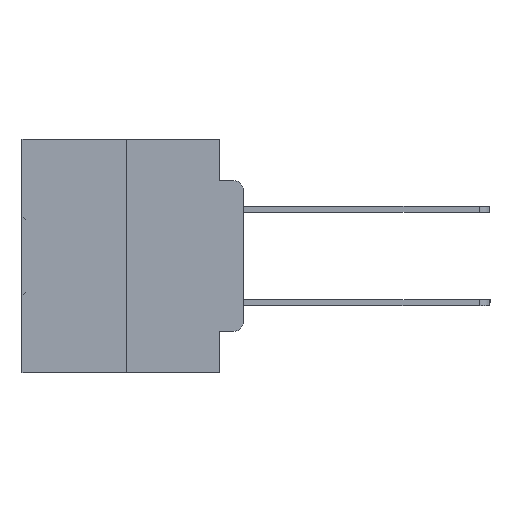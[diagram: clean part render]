
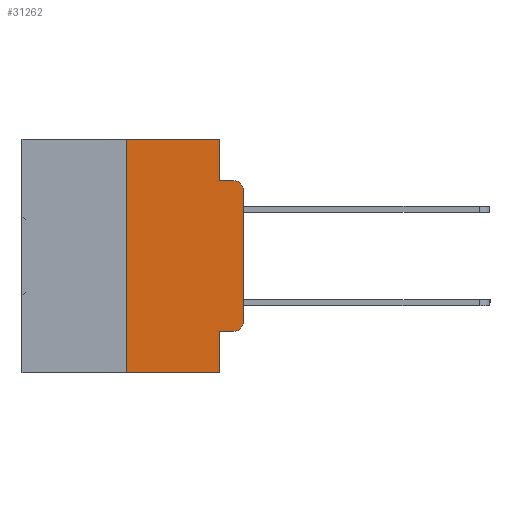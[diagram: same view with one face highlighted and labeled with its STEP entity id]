
A CAD part, left-side view. The second image highlights one B-rep face of the part: STEP entity #31262.
In plain terms, the highlighted planar face has unit normal (-1, 0, 0).
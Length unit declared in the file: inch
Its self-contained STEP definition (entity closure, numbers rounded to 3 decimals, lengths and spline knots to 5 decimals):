
#1554 = CARTESIAN_POINT ( 'NONE',  ( 0., 0.051, 0. ) ) ;
#1672 = LINE ( 'NONE', #30385, #8848 ) ;
#1958 = ORIENTED_EDGE ( 'NONE', *, *, #12884, .F. ) ;
#2787 = EDGE_CURVE ( 'NONE', #33220, #21981, #1672, .T. ) ;
#2866 = LINE ( 'NONE', #29485, #5395 ) ;
#2872 = ORIENTED_EDGE ( 'NONE', *, *, #27728, .F. ) ;
#3043 = DIRECTION ( 'NONE',  ( 0., 0., -1. ) ) ;
#3570 = AXIS2_PLACEMENT_3D ( 'NONE', #33769, #7309, #20546 ) ;
#3687 = CARTESIAN_POINT ( 'NONE',  ( 0., 0.25, -0.5 ) ) ;
#4834 = VECTOR ( 'NONE', #13525, 39.37008 ) ;
#5395 = VECTOR ( 'NONE', #16601, 39.37008 ) ;
#5457 = VERTEX_POINT ( 'NONE', #22068 ) ;
#5616 = EDGE_CURVE ( 'NONE', #27667, #25317, #27909, .T. ) ;
#6522 = AXIS2_PLACEMENT_3D ( 'NONE', #9857, #33035, #30807 ) ;
#7129 = LINE ( 'NONE', #9218, #18200 ) ;
#7202 = VECTOR ( 'NONE', #26392, 39.37008 ) ;
#7309 = DIRECTION ( 'NONE',  ( -1., 0., 0. ) ) ;
#8848 = VECTOR ( 'NONE', #17325, 39.37008 ) ;
#9218 = CARTESIAN_POINT ( 'NONE',  ( 0., 0.473, -0.5 ) ) ;
#9736 = ORIENTED_EDGE ( 'NONE', *, *, #5616, .T. ) ;
#9857 = CARTESIAN_POINT ( 'NONE',  ( 0., 0.02, -0.1085 ) ) ;
#10055 = EDGE_CURVE ( 'NONE', #10341, #11048, #20272, .T. ) ;
#10316 = ORIENTED_EDGE ( 'NONE', *, *, #2787, .F. ) ;
#10341 = VERTEX_POINT ( 'NONE', #33583 ) ;
#10538 = CARTESIAN_POINT ( 'NONE',  ( 0., 0., -0.3915 ) ) ;
#10857 = EDGE_CURVE ( 'NONE', #25317, #25106, #15859, .T. ) ;
#11048 = VERTEX_POINT ( 'NONE', #20669 ) ;
#11307 = ORIENTED_EDGE ( 'NONE', *, *, #26662, .T. ) ;
#12119 = DIRECTION ( 'NONE',  ( 0., -1., 0. ) ) ;
#12334 = VERTEX_POINT ( 'NONE', #25930 ) ;
#12884 = EDGE_CURVE ( 'NONE', #12334, #25106, #20515, .T. ) ;
#13357 = DIRECTION ( 'NONE',  ( 1., 0., 0. ) ) ;
#13525 = DIRECTION ( 'NONE',  ( 0., 0., -1. ) ) ;
#13630 = CARTESIAN_POINT ( 'NONE',  ( 0., 0.25, 0. ) ) ;
#13738 = VECTOR ( 'NONE', #19167, 39.37008 ) ;
#13755 = EDGE_CURVE ( 'NONE', #33220, #11048, #7129, .T. ) ;
#13870 = CARTESIAN_POINT ( 'NONE',  ( 0., 0.473, 0. ) ) ;
#14036 = LINE ( 'NONE', #19345, #13738 ) ;
#14799 = CARTESIAN_POINT ( 'NONE',  ( 0., 0., -0.1085 ) ) ;
#15037 = CARTESIAN_POINT ( 'NONE',  ( 0., 0., 0. ) ) ;
#15116 = ORIENTED_EDGE ( 'NONE', *, *, #22847, .F. ) ;
#15437 = LINE ( 'NONE', #20407, #7202 ) ;
#15859 = CIRCLE ( 'NONE', #6522, 0.02 ) ;
#16601 = DIRECTION ( 'NONE',  ( 0., 0., -1. ) ) ;
#17325 = DIRECTION ( 'NONE',  ( 0., 0., 1. ) ) ;
#17774 = DIRECTION ( 'NONE',  ( 0., 0., 1. ) ) ;
#18200 = VECTOR ( 'NONE', #12119, 39.37008 ) ;
#18272 = DIRECTION ( 'NONE',  ( 0., -1., 0. ) ) ;
#18820 = ORIENTED_EDGE ( 'NONE', *, *, #10055, .F. ) ;
#18857 = VECTOR ( 'NONE', #17774, 39.37008 ) ;
#19167 = DIRECTION ( 'NONE',  ( 0., -1., 0. ) ) ;
#19345 = CARTESIAN_POINT ( 'NONE',  ( 0., 0.051, -0.4115 ) ) ;
#20272 = LINE ( 'NONE', #21245, #4834 ) ;
#20318 = ORIENTED_EDGE ( 'NONE', *, *, #32811, .T. ) ;
#20407 = CARTESIAN_POINT ( 'NONE',  ( 0., 0.473, 0. ) ) ;
#20515 = LINE ( 'NONE', #25829, #26920 ) ;
#20546 = DIRECTION ( 'NONE',  ( 0., 0., -1. ) ) ;
#20669 = CARTESIAN_POINT ( 'NONE',  ( 0., 0.051, -0.5 ) ) ;
#21245 = CARTESIAN_POINT ( 'NONE',  ( 0., 0.051, 0. ) ) ;
#21323 = CARTESIAN_POINT ( 'NONE',  ( 0., 0.02, -0.0885 ) ) ;
#21405 = FACE_OUTER_BOUND ( 'NONE', #28616, .T. ) ;
#21981 = VERTEX_POINT ( 'NONE', #13630 ) ;
#22068 = CARTESIAN_POINT ( 'NONE',  ( 0., 0.02, -0.4115 ) ) ;
#22847 = EDGE_CURVE ( 'NONE', #24021, #12334, #2866, .T. ) ;
#24021 = VERTEX_POINT ( 'NONE', #1554 ) ;
#25106 = VERTEX_POINT ( 'NONE', #21323 ) ;
#25317 = VERTEX_POINT ( 'NONE', #14799 ) ;
#25829 = CARTESIAN_POINT ( 'NONE',  ( 0., 0.051, -0.0885 ) ) ;
#25930 = CARTESIAN_POINT ( 'NONE',  ( 0., 0.051, -0.0885 ) ) ;
#26392 = DIRECTION ( 'NONE',  ( 0., -1., 0. ) ) ;
#26569 = PLANE ( 'NONE',  #27619 ) ;
#26662 = EDGE_CURVE ( 'NONE', #10341, #5457, #14036, .T. ) ;
#26920 = VECTOR ( 'NONE', #18272, 39.37008 ) ;
#27619 = AXIS2_PLACEMENT_3D ( 'NONE', #13870, #13357, #3043 ) ;
#27667 = VERTEX_POINT ( 'NONE', #10538 ) ;
#27728 = EDGE_CURVE ( 'NONE', #21981, #24021, #15437, .T. ) ;
#27909 = LINE ( 'NONE', #15037, #18857 ) ;
#28616 = EDGE_LOOP ( 'NONE', ( #9736, #32737, #1958, #15116, #2872, #10316, #32905, #18820, #11307, #20318 ) ) ;
#29485 = CARTESIAN_POINT ( 'NONE',  ( 0., 0.051, 0. ) ) ;
#30385 = CARTESIAN_POINT ( 'NONE',  ( 0., 0.25, 0. ) ) ;
#30451 = CIRCLE ( 'NONE', #3570, 0.02 ) ;
#30807 = DIRECTION ( 'NONE',  ( 0., 0., -1. ) ) ;
#31262 = ADVANCED_FACE ( 'NONE', ( #21405 ), #26569, .F. ) ;
#32737 = ORIENTED_EDGE ( 'NONE', *, *, #10857, .T. ) ;
#32811 = EDGE_CURVE ( 'NONE', #5457, #27667, #30451, .T. ) ;
#32905 = ORIENTED_EDGE ( 'NONE', *, *, #13755, .T. ) ;
#33035 = DIRECTION ( 'NONE',  ( -1., 0., 0. ) ) ;
#33220 = VERTEX_POINT ( 'NONE', #3687 ) ;
#33583 = CARTESIAN_POINT ( 'NONE',  ( 0., 0.051, -0.4115 ) ) ;
#33769 = CARTESIAN_POINT ( 'NONE',  ( 0., 0.02, -0.3915 ) ) ;
